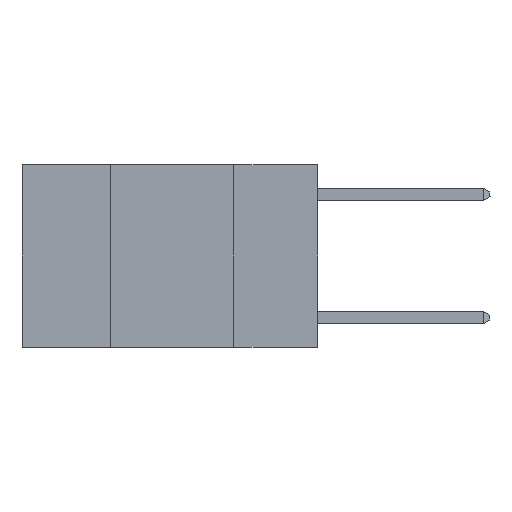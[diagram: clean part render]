
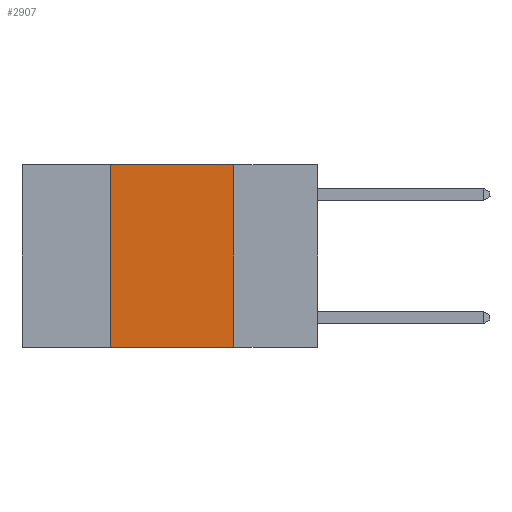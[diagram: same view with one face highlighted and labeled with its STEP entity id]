
A CAD part, left-side view. The second image highlights one B-rep face of the part: STEP entity #2907.
In plain terms, the highlighted planar face has unit normal (-1, 0, 0).
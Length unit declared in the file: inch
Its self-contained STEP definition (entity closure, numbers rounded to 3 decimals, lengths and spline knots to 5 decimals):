
#379 = CARTESIAN_POINT ( 'NONE',  ( 0., 0.42, 0. ) ) ;
#748 = EDGE_LOOP ( 'NONE', ( #7708, #6308, #4288, #4575 ) ) ;
#885 = EDGE_CURVE ( 'NONE', #3260, #8280, #2780, .T. ) ;
#932 = DIRECTION ( 'NONE',  ( 0., 0., -1. ) ) ;
#1161 = VERTEX_POINT ( 'NONE', #9714 ) ;
#1400 = CARTESIAN_POINT ( 'NONE',  ( 0., 0.6, -0.37 ) ) ;
#2128 = VECTOR ( 'NONE', #8284, 39.37008 ) ;
#2513 = DIRECTION ( 'NONE',  ( 0., 0., -1. ) ) ;
#2526 = DIRECTION ( 'NONE',  ( 1., 0., 0. ) ) ;
#2625 = PLANE ( 'NONE',  #7465 ) ;
#2634 = CARTESIAN_POINT ( 'NONE',  ( 0., 0.6, 0. ) ) ;
#2780 = LINE ( 'NONE', #10949, #9236 ) ;
#2907 = ADVANCED_FACE ( 'NONE', ( #9689 ), #2625, .F. ) ;
#3113 = CARTESIAN_POINT ( 'NONE',  ( 0., 0.42, 0. ) ) ;
#3260 = VERTEX_POINT ( 'NONE', #379 ) ;
#3998 = DIRECTION ( 'NONE',  ( 0., 0., 1. ) ) ;
#4277 = CARTESIAN_POINT ( 'NONE',  ( 0., 0.42, -0.37 ) ) ;
#4288 = ORIENTED_EDGE ( 'NONE', *, *, #4974, .F. ) ;
#4461 = LINE ( 'NONE', #1400, #2128 ) ;
#4505 = VERTEX_POINT ( 'NONE', #4277 ) ;
#4575 = ORIENTED_EDGE ( 'NONE', *, *, #5722, .T. ) ;
#4723 = EDGE_CURVE ( 'NONE', #8280, #1161, #8273, .T. ) ;
#4974 = EDGE_CURVE ( 'NONE', #4505, #3260, #10687, .T. ) ;
#5722 = EDGE_CURVE ( 'NONE', #4505, #1161, #4461, .T. ) ;
#6095 = VECTOR ( 'NONE', #932, 39.37008 ) ;
#6308 = ORIENTED_EDGE ( 'NONE', *, *, #885, .F. ) ;
#7465 = AXIS2_PLACEMENT_3D ( 'NONE', #2634, #2526, #2513 ) ;
#7708 = ORIENTED_EDGE ( 'NONE', *, *, #4723, .F. ) ;
#7880 = VECTOR ( 'NONE', #3998, 39.37008 ) ;
#8273 = LINE ( 'NONE', #10980, #6095 ) ;
#8280 = VERTEX_POINT ( 'NONE', #10815 ) ;
#8284 = DIRECTION ( 'NONE',  ( 0., -1., 0. ) ) ;
#9236 = VECTOR ( 'NONE', #9774, 39.37008 ) ;
#9689 = FACE_OUTER_BOUND ( 'NONE', #748, .T. ) ;
#9714 = CARTESIAN_POINT ( 'NONE',  ( 0., 0.17, -0.37 ) ) ;
#9774 = DIRECTION ( 'NONE',  ( 0., -1., 0. ) ) ;
#10687 = LINE ( 'NONE', #3113, #7880 ) ;
#10815 = CARTESIAN_POINT ( 'NONE',  ( 0., 0.17, 0. ) ) ;
#10949 = CARTESIAN_POINT ( 'NONE',  ( 0., 0.6, 0. ) ) ;
#10980 = CARTESIAN_POINT ( 'NONE',  ( 0., 0.17, 0. ) ) ;
